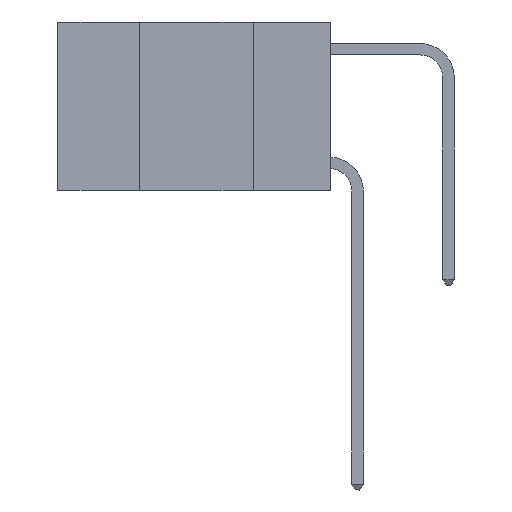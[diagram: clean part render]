
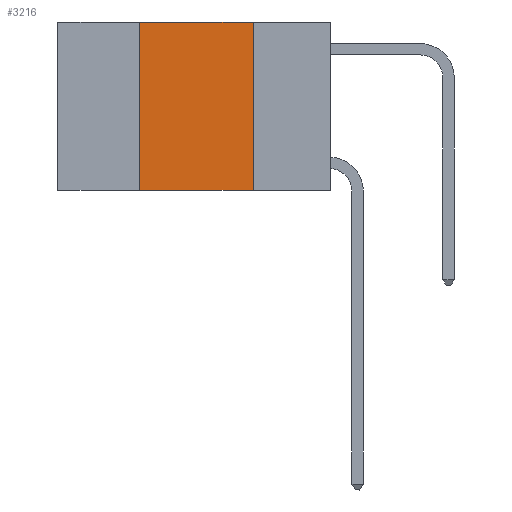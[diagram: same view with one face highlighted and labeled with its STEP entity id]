
A CAD part, left-side view. The second image highlights one B-rep face of the part: STEP entity #3216.
In plain terms, the highlighted planar face has unit normal (-1, 0, 0).
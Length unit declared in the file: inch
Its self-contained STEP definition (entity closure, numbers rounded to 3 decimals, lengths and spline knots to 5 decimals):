
#111 = LINE ( 'NONE', #11664, #10863 ) ;
#118 = CARTESIAN_POINT ( 'NONE',  ( 0., 0.6, 0. ) ) ;
#201 = DIRECTION ( 'NONE',  ( 1., 0., 0. ) ) ;
#483 = FACE_OUTER_BOUND ( 'NONE', #6720, .T. ) ;
#764 = AXIS2_PLACEMENT_3D ( 'NONE', #118, #201, #10075 ) ;
#1146 = ORIENTED_EDGE ( 'NONE', *, *, #8098, .F. ) ;
#1515 = CARTESIAN_POINT ( 'NONE',  ( 0., 0.6, -0.37 ) ) ;
#1549 = DIRECTION ( 'NONE',  ( 0., -1., 0. ) ) ;
#1920 = VERTEX_POINT ( 'NONE', #6321 ) ;
#2667 = LINE ( 'NONE', #10157, #9668 ) ;
#3144 = VECTOR ( 'NONE', #3262, 39.37008 ) ;
#3216 = ADVANCED_FACE ( 'NONE', ( #483 ), #12089, .F. ) ;
#3262 = DIRECTION ( 'NONE',  ( 0., 0., -1. ) ) ;
#3836 = LINE ( 'NONE', #1515, #5729 ) ;
#3891 = CARTESIAN_POINT ( 'NONE',  ( 0., 0.42, 0. ) ) ;
#4187 = EDGE_CURVE ( 'NONE', #10117, #1920, #3836, .T. ) ;
#5484 = DIRECTION ( 'NONE',  ( 0., -1., 0. ) ) ;
#5729 = VECTOR ( 'NONE', #5484, 39.37008 ) ;
#6321 = CARTESIAN_POINT ( 'NONE',  ( 0., 0.17, -0.37 ) ) ;
#6720 = EDGE_LOOP ( 'NONE', ( #6777, #6823, #1146, #12361 ) ) ;
#6777 = ORIENTED_EDGE ( 'NONE', *, *, #7509, .F. ) ;
#6823 = ORIENTED_EDGE ( 'NONE', *, *, #11341, .F. ) ;
#7509 = EDGE_CURVE ( 'NONE', #11411, #1920, #10642, .T. ) ;
#8098 = EDGE_CURVE ( 'NONE', #10117, #11644, #2667, .T. ) ;
#9668 = VECTOR ( 'NONE', #12335, 39.37008 ) ;
#10075 = DIRECTION ( 'NONE',  ( 0., 0., -1. ) ) ;
#10117 = VERTEX_POINT ( 'NONE', #11448 ) ;
#10157 = CARTESIAN_POINT ( 'NONE',  ( 0., 0.42, 0. ) ) ;
#10642 = LINE ( 'NONE', #12466, #3144 ) ;
#10827 = CARTESIAN_POINT ( 'NONE',  ( 0., 0.17, 0. ) ) ;
#10863 = VECTOR ( 'NONE', #1549, 39.37008 ) ;
#11341 = EDGE_CURVE ( 'NONE', #11644, #11411, #111, .T. ) ;
#11411 = VERTEX_POINT ( 'NONE', #10827 ) ;
#11448 = CARTESIAN_POINT ( 'NONE',  ( 0., 0.42, -0.37 ) ) ;
#11644 = VERTEX_POINT ( 'NONE', #3891 ) ;
#11664 = CARTESIAN_POINT ( 'NONE',  ( 0., 0.6, 0. ) ) ;
#12089 = PLANE ( 'NONE',  #764 ) ;
#12335 = DIRECTION ( 'NONE',  ( 0., 0., 1. ) ) ;
#12361 = ORIENTED_EDGE ( 'NONE', *, *, #4187, .T. ) ;
#12466 = CARTESIAN_POINT ( 'NONE',  ( 0., 0.17, 0. ) ) ;
